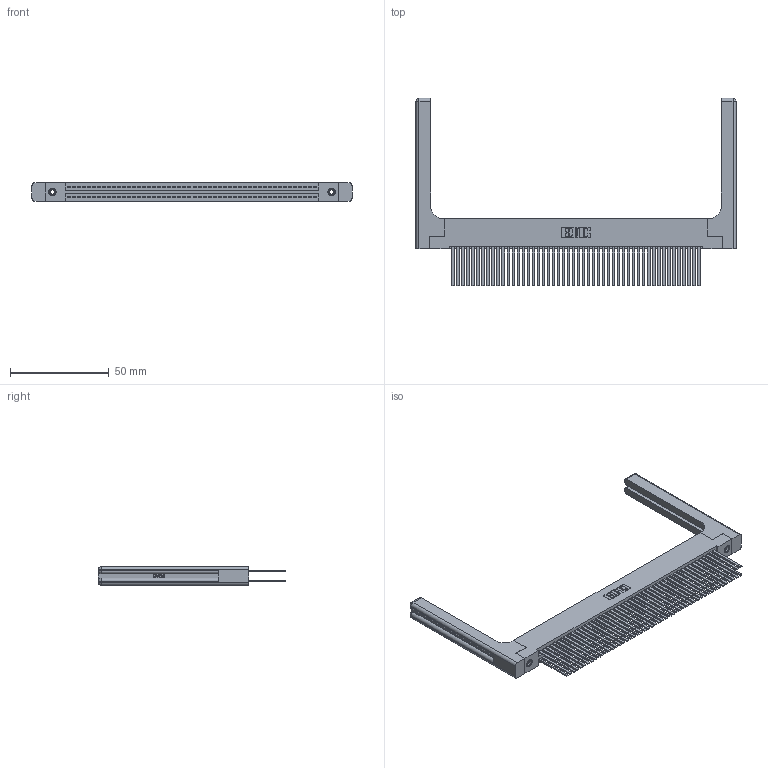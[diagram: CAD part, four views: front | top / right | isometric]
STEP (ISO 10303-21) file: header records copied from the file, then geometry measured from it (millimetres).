
FILE_DESCRIPTION (( 'STEP AP203' ), '1' );
FILE_NAME ('395-100-544-258.STEP', '2019-10-26T16:01:09', ( '' ), ( '' ), 'SwSTEP 2.0', 'SolidWorks 2016', '' );
FILE_SCHEMA (( 'CONFIG_CONTROL_DESIGN' ));
Length unit declared in the file: inch
Products named in the file (5): 345 Part_Flush Mounting Lugs - 0.156 Dia-TH; 345-292-001_345-293-144; 345-250-001_345-250-001-102; 345-220-058_345-220-058; 395-100-544-258
Assembly tree (105 placements, depth 2):
  395-100-544-258
    345 Part_Flush Mounting Lugs - 0.156 Dia-TH
    345-292-001_345-293-144  x100
    345-250-001_345-250-001-102  x2
    345-220-058_345-220-058  x2
Bounding box: 162.03 x 94.92 x 9.4 mm (x, y, z)
Volume: 25690.6 mm3; surface area: 34769.8 mm2
Topology: 105 solids, 105 shells, 4782 faces, 14107 edges, 9250 vertices
Faces by surface type: plane 3128, cylinder 1594, bspline 36, cone 12, sphere 8, torus 4
Entity records: 43152 total; most frequent: CARTESIAN_POINT 8217, ORIENTED_EDGE 6948, DIRECTION 6166, EDGE_CURVE 3474, LINE 3054, VECTOR 3054, VERTEX_POINT 2306, AXIS2_PLACEMENT_3D 1556
